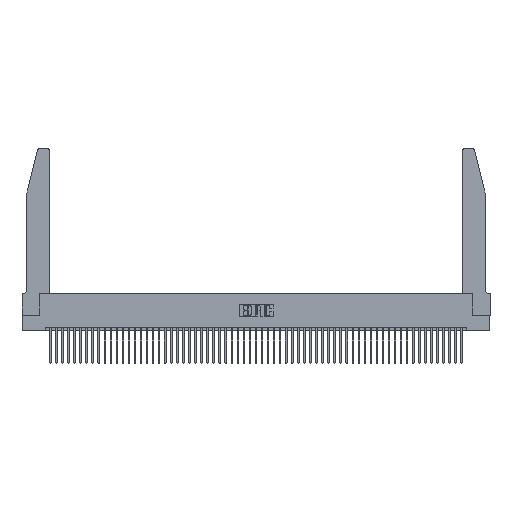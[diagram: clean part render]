
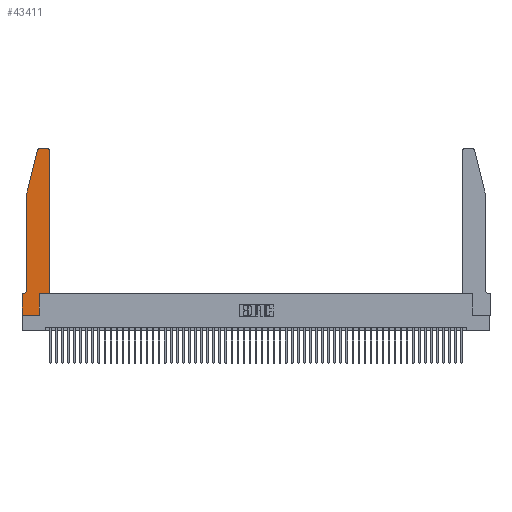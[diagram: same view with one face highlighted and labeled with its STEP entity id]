
A CAD part, top view. The second image highlights one B-rep face of the part: STEP entity #43411.
In plain terms, the highlighted planar face has unit normal (0, 0, 1).
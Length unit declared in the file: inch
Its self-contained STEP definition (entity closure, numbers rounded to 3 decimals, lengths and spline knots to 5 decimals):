
#196 = CARTESIAN_POINT ( 'NONE',  ( 0.0755, 2., 0.37 ) ) ;
#689 = VECTOR ( 'NONE', #19858, 39.37008 ) ;
#1583 = VERTEX_POINT ( 'NONE', #43667 ) ;
#1685 = EDGE_CURVE ( 'NONE', #9645, #14210, #8987, .T. ) ;
#1936 = EDGE_CURVE ( 'NONE', #39843, #52459, #27035, .T. ) ;
#1968 = LINE ( 'NONE', #36915, #689 ) ;
#2368 = LINE ( 'NONE', #27957, #9704 ) ;
#2452 = CARTESIAN_POINT ( 'NONE',  ( 0.0055, 0.35, 0.37 ) ) ;
#2610 = DIRECTION ( 'NONE',  ( 1., 0., 0. ) ) ;
#3888 = CARTESIAN_POINT ( 'NONE',  ( 0.284, 2.75, 0.37 ) ) ;
#5375 = ORIENTED_EDGE ( 'NONE', *, *, #23081, .T. ) ;
#5950 = ORIENTED_EDGE ( 'NONE', *, *, #23524, .T. ) ;
#6255 = LINE ( 'NONE', #53854, #25545 ) ;
#6478 = VERTEX_POINT ( 'NONE', #19545 ) ;
#6511 = DIRECTION ( 'NONE',  ( 0., 0., 1. ) ) ;
#6942 = DIRECTION ( 'NONE',  ( 0., 0., -1. ) ) ;
#6978 = DIRECTION ( 'NONE',  ( 0., 1., 0. ) ) ;
#6985 = ORIENTED_EDGE ( 'NONE', *, *, #41450, .T. ) ;
#7111 = CARTESIAN_POINT ( 'NONE',  ( 0.2865, 0., 0.37 ) ) ;
#7819 = EDGE_CURVE ( 'NONE', #52459, #23394, #2368, .T. ) ;
#8767 = CARTESIAN_POINT ( 'NONE',  ( 0.2605, 2.75, 0.37 ) ) ;
#8987 = CIRCLE ( 'NONE', #23572, 0.03 ) ;
#9629 = ORIENTED_EDGE ( 'NONE', *, *, #35566, .T. ) ;
#9645 = VERTEX_POINT ( 'NONE', #35848 ) ;
#9704 = VECTOR ( 'NONE', #45392, 39.37008 ) ;
#10490 = VERTEX_POINT ( 'NONE', #2452 ) ;
#11729 = VECTOR ( 'NONE', #50929, 39.37008 ) ;
#12915 = CIRCLE ( 'NONE', #20426, 0.03 ) ;
#13102 = LINE ( 'NONE', #41637, #48486 ) ;
#14093 = EDGE_CURVE ( 'NONE', #1583, #15417, #6255, .T. ) ;
#14210 = VERTEX_POINT ( 'NONE', #37556 ) ;
#15008 = LINE ( 'NONE', #8767, #11729 ) ;
#15417 = VERTEX_POINT ( 'NONE', #53533 ) ;
#16387 = DIRECTION ( 'NONE',  ( 0., -1., 0. ) ) ;
#17050 = CIRCLE ( 'NONE', #39435, 0.07 ) ;
#17478 = CARTESIAN_POINT ( 'NONE',  ( 0., 0.35, 0.37 ) ) ;
#17651 = CARTESIAN_POINT ( 'NONE',  ( 0.0755, 0.35, 0.37 ) ) ;
#18579 = CARTESIAN_POINT ( 'NONE',  ( 0.2865, 0.35, 0.37 ) ) ;
#18829 = VECTOR ( 'NONE', #49014, 39.37008 ) ;
#18976 = CARTESIAN_POINT ( 'NONE',  ( 0.284, 2.72, 0.37 ) ) ;
#19019 = VERTEX_POINT ( 'NONE', #3888 ) ;
#19195 = DIRECTION ( 'NONE',  ( -1., 0., 0. ) ) ;
#19478 = EDGE_CURVE ( 'NONE', #6478, #39843, #1968, .T. ) ;
#19545 = CARTESIAN_POINT ( 'NONE',  ( 0., 0., 0.37 ) ) ;
#19858 = DIRECTION ( 'NONE',  ( 1., 0., 0. ) ) ;
#20365 = ORIENTED_EDGE ( 'NONE', *, *, #14093, .T. ) ;
#20426 = AXIS2_PLACEMENT_3D ( 'NONE', #18976, #27721, #32412 ) ;
#20446 = CARTESIAN_POINT ( 'NONE',  ( 0., 0.35, 0.37 ) ) ;
#21471 = ORIENTED_EDGE ( 'NONE', *, *, #7819, .T. ) ;
#23081 = EDGE_CURVE ( 'NONE', #19019, #1583, #12915, .T. ) ;
#23106 = ORIENTED_EDGE ( 'NONE', *, *, #1685, .T. ) ;
#23394 = VERTEX_POINT ( 'NONE', #25796 ) ;
#23524 = EDGE_CURVE ( 'NONE', #28813, #6478, #45614, .T. ) ;
#23572 = AXIS2_PLACEMENT_3D ( 'NONE', #49069, #6511, #2610 ) ;
#25545 = VECTOR ( 'NONE', #37378, 39.37008 ) ;
#25796 = CARTESIAN_POINT ( 'NONE',  ( 0.4505, 0.35, 0.37 ) ) ;
#27035 = LINE ( 'NONE', #47138, #28321 ) ;
#27423 = VECTOR ( 'NONE', #43253, 39.37008 ) ;
#27721 = DIRECTION ( 'NONE',  ( 0., 0., 1. ) ) ;
#27957 = CARTESIAN_POINT ( 'NONE',  ( 0.4505, 0.35, 0.37 ) ) ;
#28321 = VECTOR ( 'NONE', #38195, 39.37008 ) ;
#28813 = VERTEX_POINT ( 'NONE', #20446 ) ;
#29960 = VECTOR ( 'NONE', #16387, 39.37008 ) ;
#29964 = DIRECTION ( 'NONE',  ( 0., 0., 1. ) ) ;
#30229 = ORIENTED_EDGE ( 'NONE', *, *, #1936, .T. ) ;
#30793 = EDGE_CURVE ( 'NONE', #15417, #35054, #51423, .T. ) ;
#32412 = DIRECTION ( 'NONE',  ( 1., 0., 0. ) ) ;
#32640 = ORIENTED_EDGE ( 'NONE', *, *, #46202, .T. ) ;
#34108 = PLANE ( 'NONE',  #42324 ) ;
#34168 = LINE ( 'NONE', #17651, #27423 ) ;
#34816 = EDGE_CURVE ( 'NONE', #23394, #9645, #13102, .T. ) ;
#35054 = VERTEX_POINT ( 'NONE', #39188 ) ;
#35566 = EDGE_CURVE ( 'NONE', #14210, #19019, #15008, .T. ) ;
#35848 = CARTESIAN_POINT ( 'NONE',  ( 0.4505, 2.72, 0.37 ) ) ;
#36915 = CARTESIAN_POINT ( 'NONE',  ( 0., 0., 0.37 ) ) ;
#37378 = DIRECTION ( 'NONE',  ( -0.239, -0.971, 0. ) ) ;
#37556 = CARTESIAN_POINT ( 'NONE',  ( 0.4205, 2.75, 0.37 ) ) ;
#38018 = ORIENTED_EDGE ( 'NONE', *, *, #34816, .T. ) ;
#38195 = DIRECTION ( 'NONE',  ( 0., 1., 0. ) ) ;
#39188 = CARTESIAN_POINT ( 'NONE',  ( 0.0755, 0.42, 0.37 ) ) ;
#39435 = AXIS2_PLACEMENT_3D ( 'NONE', #44822, #6942, #19195 ) ;
#39843 = VERTEX_POINT ( 'NONE', #7111 ) ;
#41450 = EDGE_CURVE ( 'NONE', #10490, #28813, #34168, .T. ) ;
#41637 = CARTESIAN_POINT ( 'NONE',  ( 0.4505, 0.35, 0.37 ) ) ;
#42324 = AXIS2_PLACEMENT_3D ( 'NONE', #17478, #29964, #43078 ) ;
#43078 = DIRECTION ( 'NONE',  ( 1., 0., 0. ) ) ;
#43253 = DIRECTION ( 'NONE',  ( -1., 0., 0. ) ) ;
#43411 = ADVANCED_FACE ( 'NONE', ( #49384 ), #34108, .T. ) ;
#43641 = ORIENTED_EDGE ( 'NONE', *, *, #30793, .T. ) ;
#43667 = CARTESIAN_POINT ( 'NONE',  ( 0.25487, 2.72718, 0.37 ) ) ;
#44352 = CARTESIAN_POINT ( 'NONE',  ( 0., 0., 0.37 ) ) ;
#44822 = CARTESIAN_POINT ( 'NONE',  ( 0.0055, 0.42, 0.37 ) ) ;
#45392 = DIRECTION ( 'NONE',  ( 1., 0., 0. ) ) ;
#45614 = LINE ( 'NONE', #44352, #18829 ) ;
#46202 = EDGE_CURVE ( 'NONE', #35054, #10490, #17050, .T. ) ;
#47138 = CARTESIAN_POINT ( 'NONE',  ( 0.2865, 0.35, 0.37 ) ) ;
#48486 = VECTOR ( 'NONE', #6978, 39.37008 ) ;
#49014 = DIRECTION ( 'NONE',  ( 0., -1., 0. ) ) ;
#49069 = CARTESIAN_POINT ( 'NONE',  ( 0.4205, 2.72, 0.37 ) ) ;
#49384 = FACE_OUTER_BOUND ( 'NONE', #51294, .T. ) ;
#50929 = DIRECTION ( 'NONE',  ( -1., 0., 0. ) ) ;
#51294 = EDGE_LOOP ( 'NONE', ( #9629, #5375, #20365, #43641, #32640, #6985, #5950, #52937, #30229, #21471, #38018, #23106 ) ) ;
#51423 = LINE ( 'NONE', #196, #29960 ) ;
#52459 = VERTEX_POINT ( 'NONE', #18579 ) ;
#52937 = ORIENTED_EDGE ( 'NONE', *, *, #19478, .T. ) ;
#53533 = CARTESIAN_POINT ( 'NONE',  ( 0.0755, 2., 0.37 ) ) ;
#53854 = CARTESIAN_POINT ( 'NONE',  ( 0.0755, 2., 0.37 ) ) ;
